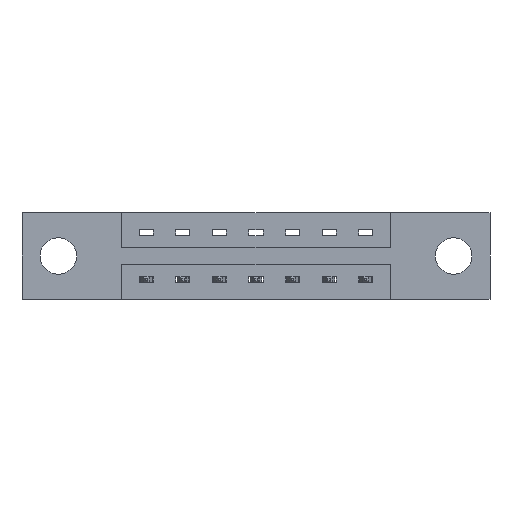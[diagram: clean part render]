
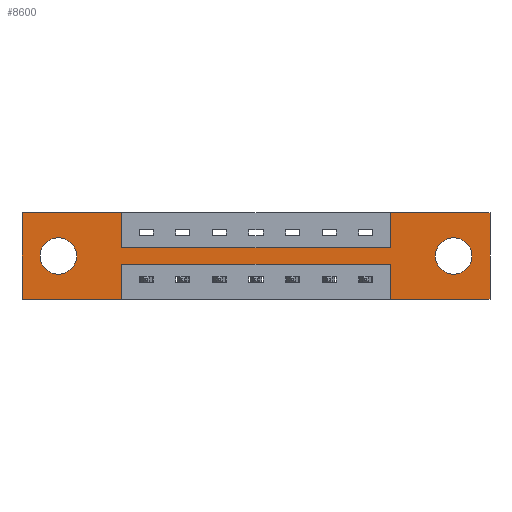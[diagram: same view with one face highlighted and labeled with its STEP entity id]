
A CAD part, front view. The second image highlights one B-rep face of the part: STEP entity #8600.
In plain terms, the highlighted planar face has unit normal (0, -1, 0).
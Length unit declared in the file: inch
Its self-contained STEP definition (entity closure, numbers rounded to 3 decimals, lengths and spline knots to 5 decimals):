
#85 = EDGE_CURVE ( 'NONE', #2784, #7350, #8836, .T. ) ;
#383 = DIRECTION ( 'NONE',  ( -1., 0., 0. ) ) ;
#606 = CARTESIAN_POINT ( 'NONE',  ( 0.155, 0., -0.107 ) ) ;
#627 = AXIS2_PLACEMENT_3D ( 'NONE', #5259, #2204, #7444 ) ;
#662 = VERTEX_POINT ( 'NONE', #7419 ) ;
#669 = CARTESIAN_POINT ( 'NONE',  ( 1.843, 0., -0.107 ) ) ;
#805 = DIRECTION ( 'NONE',  ( -1., 0., 0. ) ) ;
#1202 = CARTESIAN_POINT ( 'NONE',  ( 1.573, 0., 0. ) ) ;
#1218 = CARTESIAN_POINT ( 'NONE',  ( 1.843, 0., -0.185 ) ) ;
#1263 = VECTOR ( 'NONE', #3616, 39.37008 ) ;
#1709 = VERTEX_POINT ( 'NONE', #6995 ) ;
#1818 = EDGE_LOOP ( 'NONE', ( #3569, #4400, #4451, #4582, #4594, #5108, #5432, #5444, #5679, #5699, #6273, #7095 ) ) ;
#1937 = EDGE_CURVE ( 'NONE', #3475, #7741, #2868, .T. ) ;
#2024 = VERTEX_POINT ( 'NONE', #2589 ) ;
#2077 = ORIENTED_EDGE ( 'NONE', *, *, #5261, .T. ) ;
#2093 = LINE ( 'NONE', #9277, #3908 ) ;
#2115 = CARTESIAN_POINT ( 'NONE',  ( 1.573, 0., 0. ) ) ;
#2196 = CIRCLE ( 'NONE', #8745, 0.078 ) ;
#2204 = DIRECTION ( 'NONE',  ( 0., -1., 0. ) ) ;
#2227 = AXIS2_PLACEMENT_3D ( 'NONE', #6354, #8526, #8974 ) ;
#2277 = ORIENTED_EDGE ( 'NONE', *, *, #6255, .T. ) ;
#2328 = LINE ( 'NONE', #7585, #8042 ) ;
#2395 = DIRECTION ( 'NONE',  ( 0., 0., 1. ) ) ;
#2429 = CARTESIAN_POINT ( 'NONE',  ( 0., 0., 0. ) ) ;
#2586 = VECTOR ( 'NONE', #805, 39.37008 ) ;
#2589 = CARTESIAN_POINT ( 'NONE',  ( 1.843, 0., -0.263 ) ) ;
#2679 = ORIENTED_EDGE ( 'NONE', *, *, #5269, .T. ) ;
#2776 = EDGE_LOOP ( 'NONE', ( #2077, #2277 ) ) ;
#2784 = VERTEX_POINT ( 'NONE', #3294 ) ;
#2826 = LINE ( 'NONE', #8127, #8474 ) ;
#2868 = CIRCLE ( 'NONE', #2227, 0.078 ) ;
#3000 = ORIENTED_EDGE ( 'NONE', *, *, #1937, .T. ) ;
#3066 = LINE ( 'NONE', #2115, #9601 ) ;
#3109 = DIRECTION ( 'NONE',  ( 1., 0., 0. ) ) ;
#3269 = VERTEX_POINT ( 'NONE', #8309 ) ;
#3294 = CARTESIAN_POINT ( 'NONE',  ( 0., 0., 0. ) ) ;
#3310 = DIRECTION ( 'NONE',  ( 1., 0., 0. ) ) ;
#3420 = EDGE_CURVE ( 'NONE', #3466, #7861, #6503, .T. ) ;
#3423 = AXIS2_PLACEMENT_3D ( 'NONE', #1218, #7765, #3738 ) ;
#3426 = CARTESIAN_POINT ( 'NONE',  ( 1.573, 0., -0.15 ) ) ;
#3466 = VERTEX_POINT ( 'NONE', #1202 ) ;
#3475 = VERTEX_POINT ( 'NONE', #4023 ) ;
#3527 = EDGE_LOOP ( 'NONE', ( #2679, #3000 ) ) ;
#3545 = CIRCLE ( 'NONE', #4959, 0.078 ) ;
#3569 = ORIENTED_EDGE ( 'NONE', *, *, #5329, .F. ) ;
#3570 = CARTESIAN_POINT ( 'NONE',  ( 0.425, 0., 0. ) ) ;
#3616 = DIRECTION ( 'NONE',  ( 0., 0., -1. ) ) ;
#3738 = DIRECTION ( 'NONE',  ( 0., 0., -1. ) ) ;
#3908 = VECTOR ( 'NONE', #3310, 39.37008 ) ;
#3952 = CARTESIAN_POINT ( 'NONE',  ( 0., 0., -0.37 ) ) ;
#4023 = CARTESIAN_POINT ( 'NONE',  ( 0.155, 0., -0.263 ) ) ;
#4031 = VERTEX_POINT ( 'NONE', #7639 ) ;
#4400 = ORIENTED_EDGE ( 'NONE', *, *, #5346, .F. ) ;
#4422 = CARTESIAN_POINT ( 'NONE',  ( 0., 0., -0.37 ) ) ;
#4451 = ORIENTED_EDGE ( 'NONE', *, *, #5362, .F. ) ;
#4582 = ORIENTED_EDGE ( 'NONE', *, *, #5137, .F. ) ;
#4594 = ORIENTED_EDGE ( 'NONE', *, *, #4911, .F. ) ;
#4610 = DIRECTION ( 'NONE',  ( 0., 1., 0. ) ) ;
#4643 = LINE ( 'NONE', #8695, #2586 ) ;
#4651 = CARTESIAN_POINT ( 'NONE',  ( 0.155, 0., -0.185 ) ) ;
#4656 = VERTEX_POINT ( 'NONE', #6061 ) ;
#4738 = EDGE_CURVE ( 'NONE', #3269, #2784, #8907, .T. ) ;
#4820 = FACE_BOUND ( 'NONE', #2776, .T. ) ;
#4911 = EDGE_CURVE ( 'NONE', #7861, #4656, #9611, .T. ) ;
#4959 = AXIS2_PLACEMENT_3D ( 'NONE', #4651, #7878, #2395 ) ;
#4985 = CARTESIAN_POINT ( 'NONE',  ( 0.425, 0., 0. ) ) ;
#5006 = VECTOR ( 'NONE', #5897, 39.37008 ) ;
#5108 = ORIENTED_EDGE ( 'NONE', *, *, #3420, .F. ) ;
#5137 = EDGE_CURVE ( 'NONE', #4656, #1709, #8803, .T. ) ;
#5181 = EDGE_CURVE ( 'NONE', #6392, #3269, #9715, .T. ) ;
#5259 = CARTESIAN_POINT ( 'NONE',  ( 0., 0., -0.37 ) ) ;
#5261 = EDGE_CURVE ( 'NONE', #8867, #2024, #7033, .T. ) ;
#5269 = EDGE_CURVE ( 'NONE', #7741, #3475, #3545, .T. ) ;
#5329 = EDGE_CURVE ( 'NONE', #6075, #6392, #2826, .T. ) ;
#5346 = EDGE_CURVE ( 'NONE', #4031, #6075, #4643, .T. ) ;
#5362 = EDGE_CURVE ( 'NONE', #1709, #4031, #2328, .T. ) ;
#5376 = EDGE_CURVE ( 'NONE', #9238, #3466, #3066, .T. ) ;
#5401 = EDGE_CURVE ( 'NONE', #662, #9238, #2093, .T. ) ;
#5413 = CARTESIAN_POINT ( 'NONE',  ( 1.998, 0., 0. ) ) ;
#5432 = ORIENTED_EDGE ( 'NONE', *, *, #5376, .F. ) ;
#5444 = ORIENTED_EDGE ( 'NONE', *, *, #5401, .F. ) ;
#5482 = CARTESIAN_POINT ( 'NONE',  ( 1.998, 0., 0. ) ) ;
#5587 = EDGE_CURVE ( 'NONE', #7350, #662, #9207, .T. ) ;
#5679 = ORIENTED_EDGE ( 'NONE', *, *, #5587, .F. ) ;
#5699 = ORIENTED_EDGE ( 'NONE', *, *, #85, .F. ) ;
#5879 = DIRECTION ( 'NONE',  ( 0., 0., -1. ) ) ;
#5889 = FACE_OUTER_BOUND ( 'NONE', #1818, .T. ) ;
#5897 = DIRECTION ( 'NONE',  ( 1., 0., 0. ) ) ;
#5981 = PLANE ( 'NONE',  #627 ) ;
#6061 = CARTESIAN_POINT ( 'NONE',  ( 1.998, 0., -0.37 ) ) ;
#6075 = VERTEX_POINT ( 'NONE', #8673 ) ;
#6255 = EDGE_CURVE ( 'NONE', #2024, #8867, #2196, .T. ) ;
#6273 = ORIENTED_EDGE ( 'NONE', *, *, #4738, .F. ) ;
#6354 = CARTESIAN_POINT ( 'NONE',  ( 0.155, 0., -0.185 ) ) ;
#6385 = VECTOR ( 'NONE', #5879, 39.37008 ) ;
#6392 = VERTEX_POINT ( 'NONE', #6974 ) ;
#6503 = LINE ( 'NONE', #2429, #5006 ) ;
#6752 = VECTOR ( 'NONE', #3109, 39.37008 ) ;
#6974 = CARTESIAN_POINT ( 'NONE',  ( 0.425, 0., -0.37 ) ) ;
#6995 = CARTESIAN_POINT ( 'NONE',  ( 1.573, 0., -0.37 ) ) ;
#7033 = CIRCLE ( 'NONE', #3423, 0.078 ) ;
#7095 = ORIENTED_EDGE ( 'NONE', *, *, #5181, .F. ) ;
#7314 = CARTESIAN_POINT ( 'NONE',  ( 0., 0., 0. ) ) ;
#7350 = VERTEX_POINT ( 'NONE', #4985 ) ;
#7419 = CARTESIAN_POINT ( 'NONE',  ( 0.425, 0., -0.15 ) ) ;
#7444 = DIRECTION ( 'NONE',  ( 0., 0., -1. ) ) ;
#7585 = CARTESIAN_POINT ( 'NONE',  ( 1.573, 0., -0.37 ) ) ;
#7639 = CARTESIAN_POINT ( 'NONE',  ( 1.573, 0., -0.22 ) ) ;
#7722 = DIRECTION ( 'NONE',  ( -1., 0., 0. ) ) ;
#7741 = VERTEX_POINT ( 'NONE', #606 ) ;
#7765 = DIRECTION ( 'NONE',  ( 0., 1., 0. ) ) ;
#7822 = DIRECTION ( 'NONE',  ( 0., 0., 1. ) ) ;
#7845 = DIRECTION ( 'NONE',  ( 0., 0., 1. ) ) ;
#7861 = VERTEX_POINT ( 'NONE', #5482 ) ;
#7878 = DIRECTION ( 'NONE',  ( 0., 1., 0. ) ) ;
#8042 = VECTOR ( 'NONE', #7822, 39.37008 ) ;
#8127 = CARTESIAN_POINT ( 'NONE',  ( 0.425, 0., -0.37 ) ) ;
#8153 = VECTOR ( 'NONE', #7722, 39.37008 ) ;
#8309 = CARTESIAN_POINT ( 'NONE',  ( 0., 0., -0.37 ) ) ;
#8360 = DIRECTION ( 'NONE',  ( 0., 0., -1. ) ) ;
#8474 = VECTOR ( 'NONE', #8360, 39.37008 ) ;
#8526 = DIRECTION ( 'NONE',  ( 0., 1., 0. ) ) ;
#8600 = ADVANCED_FACE ( 'NONE', ( #4820, #9359, #5889 ), #5981, .T. ) ;
#8673 = CARTESIAN_POINT ( 'NONE',  ( 0.425, 0., -0.22 ) ) ;
#8695 = CARTESIAN_POINT ( 'NONE',  ( 0.425, 0., -0.22 ) ) ;
#8745 = AXIS2_PLACEMENT_3D ( 'NONE', #8902, #4610, #9548 ) ;
#8803 = LINE ( 'NONE', #3952, #8153 ) ;
#8836 = LINE ( 'NONE', #9289, #6752 ) ;
#8863 = DIRECTION ( 'NONE',  ( 0., 0., 1. ) ) ;
#8867 = VERTEX_POINT ( 'NONE', #669 ) ;
#8902 = CARTESIAN_POINT ( 'NONE',  ( 1.843, 0., -0.185 ) ) ;
#8907 = LINE ( 'NONE', #7314, #9310 ) ;
#8974 = DIRECTION ( 'NONE',  ( 0., 0., 1. ) ) ;
#9207 = LINE ( 'NONE', #3570, #1263 ) ;
#9238 = VERTEX_POINT ( 'NONE', #3426 ) ;
#9277 = CARTESIAN_POINT ( 'NONE',  ( 0.425, 0., -0.15 ) ) ;
#9289 = CARTESIAN_POINT ( 'NONE',  ( 0., 0., 0. ) ) ;
#9310 = VECTOR ( 'NONE', #7845, 39.37008 ) ;
#9359 = FACE_BOUND ( 'NONE', #3527, .T. ) ;
#9504 = VECTOR ( 'NONE', #383, 39.37008 ) ;
#9548 = DIRECTION ( 'NONE',  ( 0., 0., -1. ) ) ;
#9601 = VECTOR ( 'NONE', #8863, 39.37008 ) ;
#9611 = LINE ( 'NONE', #5413, #6385 ) ;
#9715 = LINE ( 'NONE', #4422, #9504 ) ;
